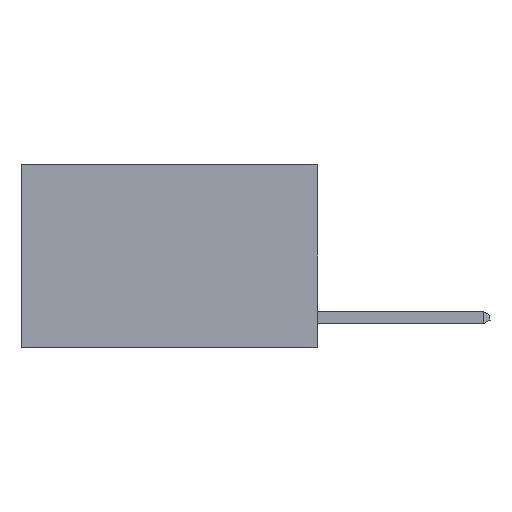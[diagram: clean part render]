
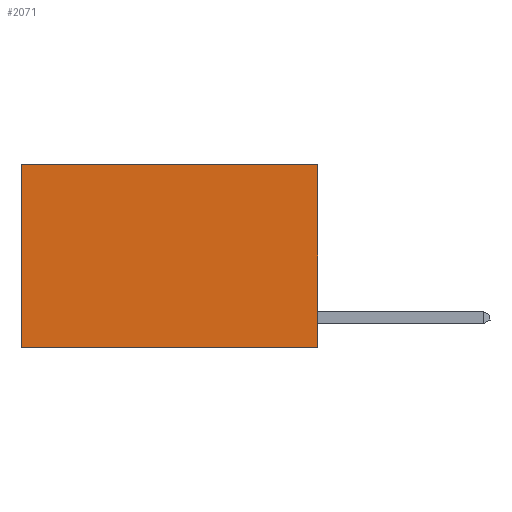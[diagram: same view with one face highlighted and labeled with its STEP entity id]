
A CAD part, left-side view. The second image highlights one B-rep face of the part: STEP entity #2071.
In plain terms, the highlighted planar face has unit normal (-1, 0, 0).
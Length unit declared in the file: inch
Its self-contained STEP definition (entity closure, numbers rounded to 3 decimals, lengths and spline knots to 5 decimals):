
#67 = EDGE_CURVE ( 'NONE', #21151, #21164, #14742, .T. ) ;
#679 = FACE_OUTER_BOUND ( 'NONE', #6532, .T. ) ;
#1072 = VECTOR ( 'NONE', #20877, 39.37008 ) ;
#1085 = VERTEX_POINT ( 'NONE', #13963 ) ;
#1691 = AXIS2_PLACEMENT_3D ( 'NONE', #3316, #19165, #6298 ) ;
#1780 = DIRECTION ( 'NONE',  ( 0., 1., 0. ) ) ;
#2071 = ADVANCED_FACE ( 'NONE', ( #679 ), #5518, .F. ) ;
#3316 = CARTESIAN_POINT ( 'NONE',  ( 0.2625, 0., 0. ) ) ;
#4553 = CARTESIAN_POINT ( 'NONE',  ( 0.2625, 0.6, -0.37 ) ) ;
#4634 = EDGE_CURVE ( 'NONE', #11838, #1085, #10080, .T. ) ;
#5079 = EDGE_CURVE ( 'NONE', #1085, #21164, #15065, .T. ) ;
#5518 = PLANE ( 'NONE',  #1691 ) ;
#5589 = VECTOR ( 'NONE', #6885, 39.37008 ) ;
#5816 = ORIENTED_EDGE ( 'NONE', *, *, #5079, .F. ) ;
#6166 = CARTESIAN_POINT ( 'NONE',  ( 0.2625, 0.6, 0. ) ) ;
#6298 = DIRECTION ( 'NONE',  ( 0., 0., -1. ) ) ;
#6532 = EDGE_LOOP ( 'NONE', ( #19856, #5816, #7364, #7930 ) ) ;
#6696 = LINE ( 'NONE', #11898, #10677 ) ;
#6885 = DIRECTION ( 'NONE',  ( 0., 1., 0. ) ) ;
#7364 = ORIENTED_EDGE ( 'NONE', *, *, #4634, .F. ) ;
#7672 = DIRECTION ( 'NONE',  ( 0., 0., -1. ) ) ;
#7930 = ORIENTED_EDGE ( 'NONE', *, *, #9855, .T. ) ;
#8511 = CARTESIAN_POINT ( 'NONE',  ( 0.2625, 0., -0.37 ) ) ;
#9855 = EDGE_CURVE ( 'NONE', #11838, #21151, #6696, .T. ) ;
#10080 = LINE ( 'NONE', #10746, #1072 ) ;
#10677 = VECTOR ( 'NONE', #1780, 39.37008 ) ;
#10746 = CARTESIAN_POINT ( 'NONE',  ( 0.2625, 0., 0. ) ) ;
#11838 = VERTEX_POINT ( 'NONE', #12332 ) ;
#11898 = CARTESIAN_POINT ( 'NONE',  ( 0.2625, 0., 0. ) ) ;
#12332 = CARTESIAN_POINT ( 'NONE',  ( 0.2625, 0., 0. ) ) ;
#13668 = CARTESIAN_POINT ( 'NONE',  ( 0.2625, 0.6, 0. ) ) ;
#13963 = CARTESIAN_POINT ( 'NONE',  ( 0.2625, 0., -0.37 ) ) ;
#14742 = LINE ( 'NONE', #13668, #18223 ) ;
#15065 = LINE ( 'NONE', #8511, #5589 ) ;
#18223 = VECTOR ( 'NONE', #7672, 39.37008 ) ;
#19165 = DIRECTION ( 'NONE',  ( 1., 0., 0. ) ) ;
#19856 = ORIENTED_EDGE ( 'NONE', *, *, #67, .T. ) ;
#20877 = DIRECTION ( 'NONE',  ( 0., 0., -1. ) ) ;
#21151 = VERTEX_POINT ( 'NONE', #6166 ) ;
#21164 = VERTEX_POINT ( 'NONE', #4553 ) ;
